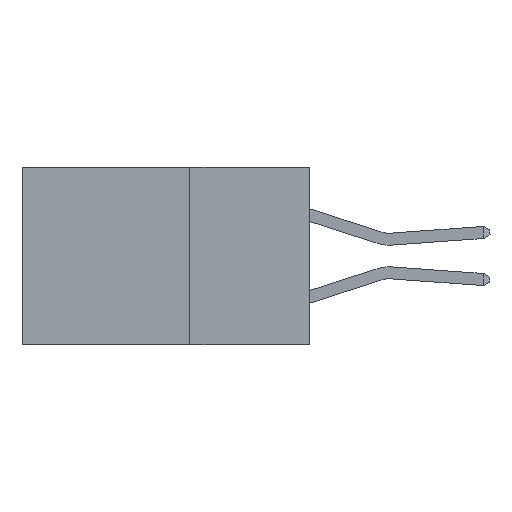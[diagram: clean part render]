
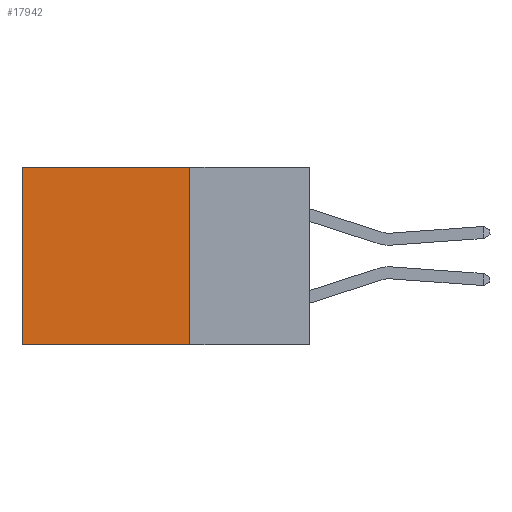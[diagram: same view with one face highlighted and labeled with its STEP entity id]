
A CAD part, left-side view. The second image highlights one B-rep face of the part: STEP entity #17942.
In plain terms, the highlighted planar face has unit normal (-1, 0, 0).
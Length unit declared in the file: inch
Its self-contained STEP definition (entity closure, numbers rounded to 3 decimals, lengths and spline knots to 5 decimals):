
#111 = DIRECTION ( 'NONE',  ( 0., 1., 0. ) ) ;
#291 = CARTESIAN_POINT ( 'NONE',  ( 0.298, 0.25, 0. ) ) ;
#461 = ORIENTED_EDGE ( 'NONE', *, *, #971, .F. ) ;
#937 = ORIENTED_EDGE ( 'NONE', *, *, #17725, .T. ) ;
#971 = EDGE_CURVE ( 'NONE', #14277, #3771, #8381, .T. ) ;
#2346 = CARTESIAN_POINT ( 'NONE',  ( 0.298, 0.25, 0. ) ) ;
#2387 = VERTEX_POINT ( 'NONE', #7269 ) ;
#3771 = VERTEX_POINT ( 'NONE', #4959 ) ;
#4039 = PLANE ( 'NONE',  #16351 ) ;
#4256 = VERTEX_POINT ( 'NONE', #8099 ) ;
#4959 = CARTESIAN_POINT ( 'NONE',  ( 0.298, 0.25, -0.37 ) ) ;
#6842 = VECTOR ( 'NONE', #111, 39.37008 ) ;
#7269 = CARTESIAN_POINT ( 'NONE',  ( 0.298, 0.6, 0. ) ) ;
#7491 = VECTOR ( 'NONE', #15442, 39.37008 ) ;
#7636 = CARTESIAN_POINT ( 'NONE',  ( 0.298, 0.25, -0.37 ) ) ;
#8099 = CARTESIAN_POINT ( 'NONE',  ( 0.298, 0.6, -0.37 ) ) ;
#8104 = ORIENTED_EDGE ( 'NONE', *, *, #12841, .F. ) ;
#8381 = LINE ( 'NONE', #10041, #19019 ) ;
#8601 = DIRECTION ( 'NONE',  ( 1., 0., 0. ) ) ;
#9701 = LINE ( 'NONE', #2346, #14575 ) ;
#10041 = CARTESIAN_POINT ( 'NONE',  ( 0.298, 0.25, 0. ) ) ;
#10355 = FACE_OUTER_BOUND ( 'NONE', #12483, .T. ) ;
#11564 = LINE ( 'NONE', #18180, #7491 ) ;
#11600 = CARTESIAN_POINT ( 'NONE',  ( 0.298, 0.25, 0. ) ) ;
#11918 = DIRECTION ( 'NONE',  ( 0., 0., -1. ) ) ;
#12483 = EDGE_LOOP ( 'NONE', ( #937, #8104, #461, #12994 ) ) ;
#12841 = EDGE_CURVE ( 'NONE', #3771, #4256, #18923, .T. ) ;
#12869 = DIRECTION ( 'NONE',  ( 0., 1., 0. ) ) ;
#12994 = ORIENTED_EDGE ( 'NONE', *, *, #13154, .T. ) ;
#13154 = EDGE_CURVE ( 'NONE', #14277, #2387, #9701, .T. ) ;
#14277 = VERTEX_POINT ( 'NONE', #291 ) ;
#14575 = VECTOR ( 'NONE', #12869, 39.37008 ) ;
#15442 = DIRECTION ( 'NONE',  ( 0., 0., -1. ) ) ;
#16351 = AXIS2_PLACEMENT_3D ( 'NONE', #11600, #8601, #18746 ) ;
#17725 = EDGE_CURVE ( 'NONE', #2387, #4256, #11564, .T. ) ;
#17942 = ADVANCED_FACE ( 'NONE', ( #10355 ), #4039, .F. ) ;
#18180 = CARTESIAN_POINT ( 'NONE',  ( 0.298, 0.6, 0. ) ) ;
#18746 = DIRECTION ( 'NONE',  ( 0., 0., -1. ) ) ;
#18923 = LINE ( 'NONE', #7636, #6842 ) ;
#19019 = VECTOR ( 'NONE', #11918, 39.37008 ) ;
